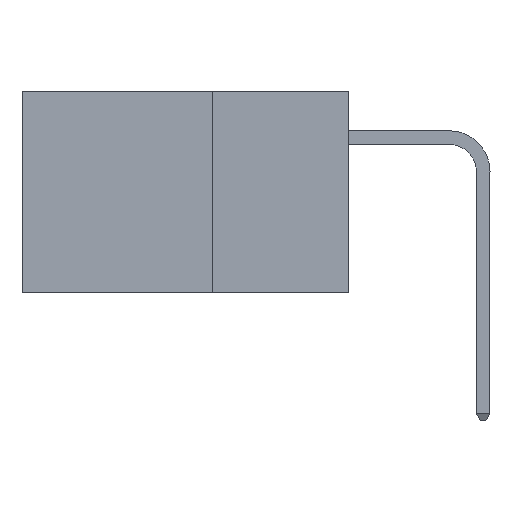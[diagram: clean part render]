
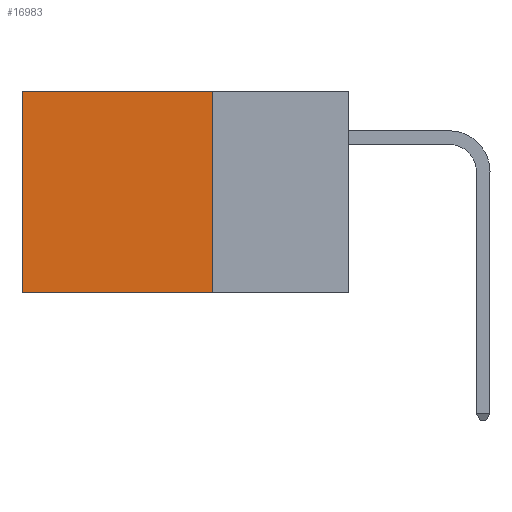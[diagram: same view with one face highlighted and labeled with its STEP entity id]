
A CAD part, left-side view. The second image highlights one B-rep face of the part: STEP entity #16983.
In plain terms, the highlighted planar face has unit normal (-1, 0, 0).
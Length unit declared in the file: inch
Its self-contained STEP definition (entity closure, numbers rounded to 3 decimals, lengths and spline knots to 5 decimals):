
#355 = VERTEX_POINT ( 'NONE', #1068 ) ;
#443 = EDGE_CURVE ( 'NONE', #23193, #23579, #13321, .T. ) ;
#567 = DIRECTION ( 'NONE',  ( 0., 0., -1. ) ) ;
#753 = LINE ( 'NONE', #1182, #5893 ) ;
#943 = FACE_OUTER_BOUND ( 'NONE', #3743, .T. ) ;
#1068 = CARTESIAN_POINT ( 'NONE',  ( 0.2875, 0.25, -0.37 ) ) ;
#1182 = CARTESIAN_POINT ( 'NONE',  ( 0.2875, 0.25, -0.37 ) ) ;
#1341 = ORIENTED_EDGE ( 'NONE', *, *, #24358, .F. ) ;
#1898 = ORIENTED_EDGE ( 'NONE', *, *, #5095, .F. ) ;
#2676 = LINE ( 'NONE', #16714, #11606 ) ;
#2950 = ORIENTED_EDGE ( 'NONE', *, *, #443, .T. ) ;
#3507 = ORIENTED_EDGE ( 'NONE', *, *, #6431, .T. ) ;
#3743 = EDGE_LOOP ( 'NONE', ( #3507, #1898, #1341, #2950 ) ) ;
#3791 = CARTESIAN_POINT ( 'NONE',  ( 0.2875, 0.6, -0.37 ) ) ;
#4169 = CARTESIAN_POINT ( 'NONE',  ( 0.2875, 0.6, 0. ) ) ;
#5095 = EDGE_CURVE ( 'NONE', #355, #7586, #753, .T. ) ;
#5573 = VECTOR ( 'NONE', #19072, 39.37008 ) ;
#5893 = VECTOR ( 'NONE', #20388, 39.37008 ) ;
#6100 = DIRECTION ( 'NONE',  ( 0., 0., -1. ) ) ;
#6431 = EDGE_CURVE ( 'NONE', #23579, #7586, #2676, .T. ) ;
#6893 = AXIS2_PLACEMENT_3D ( 'NONE', #17683, #25941, #13592 ) ;
#7141 = PLANE ( 'NONE',  #6893 ) ;
#7586 = VERTEX_POINT ( 'NONE', #3791 ) ;
#11606 = VECTOR ( 'NONE', #6100, 39.37008 ) ;
#13321 = LINE ( 'NONE', #20901, #5573 ) ;
#13592 = DIRECTION ( 'NONE',  ( 0., 0., -1. ) ) ;
#16691 = LINE ( 'NONE', #17716, #22153 ) ;
#16714 = CARTESIAN_POINT ( 'NONE',  ( 0.2875, 0.6, 0. ) ) ;
#16983 = ADVANCED_FACE ( 'NONE', ( #943 ), #7141, .F. ) ;
#17683 = CARTESIAN_POINT ( 'NONE',  ( 0.2875, 0.25, 0. ) ) ;
#17716 = CARTESIAN_POINT ( 'NONE',  ( 0.2875, 0.25, 0. ) ) ;
#19072 = DIRECTION ( 'NONE',  ( 0., 1., 0. ) ) ;
#20388 = DIRECTION ( 'NONE',  ( 0., 1., 0. ) ) ;
#20901 = CARTESIAN_POINT ( 'NONE',  ( 0.2875, 0.25, 0. ) ) ;
#22153 = VECTOR ( 'NONE', #567, 39.37008 ) ;
#23193 = VERTEX_POINT ( 'NONE', #23867 ) ;
#23579 = VERTEX_POINT ( 'NONE', #4169 ) ;
#23867 = CARTESIAN_POINT ( 'NONE',  ( 0.2875, 0.25, 0. ) ) ;
#24358 = EDGE_CURVE ( 'NONE', #23193, #355, #16691, .T. ) ;
#25941 = DIRECTION ( 'NONE',  ( 1., 0., 0. ) ) ;
